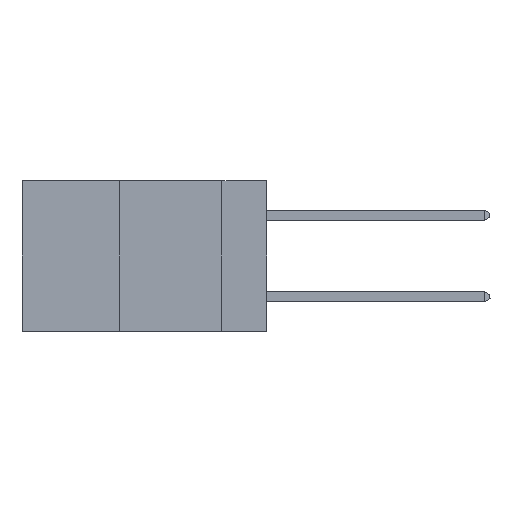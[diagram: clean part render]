
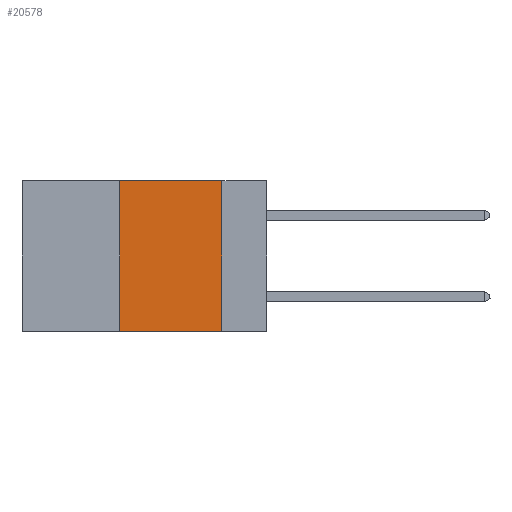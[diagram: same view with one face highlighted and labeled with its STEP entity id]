
A CAD part, left-side view. The second image highlights one B-rep face of the part: STEP entity #20578.
In plain terms, the highlighted planar face has unit normal (-1, 0, 0).
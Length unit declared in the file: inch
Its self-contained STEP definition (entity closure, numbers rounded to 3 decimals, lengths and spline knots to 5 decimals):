
#729 = VECTOR ( 'NONE', #40134, 39.37008 ) ;
#1886 = DIRECTION ( 'NONE',  ( 1., 0., 0. ) ) ;
#1929 = ORIENTED_EDGE ( 'NONE', *, *, #42733, .F. ) ;
#3078 = DIRECTION ( 'NONE',  ( 0., 0., 1. ) ) ;
#4590 = CARTESIAN_POINT ( 'NONE',  ( 0., 0.11, 0. ) ) ;
#6952 = FACE_OUTER_BOUND ( 'NONE', #26723, .T. ) ;
#14040 = EDGE_CURVE ( 'NONE', #44222, #44267, #23990, .T. ) ;
#16548 = PLANE ( 'NONE',  #31509 ) ;
#16716 = CARTESIAN_POINT ( 'NONE',  ( 0., 0.36, -0.37 ) ) ;
#18320 = DIRECTION ( 'NONE',  ( 0., 0., -1. ) ) ;
#20578 = ADVANCED_FACE ( 'NONE', ( #6952 ), #16548, .F. ) ;
#22986 = VERTEX_POINT ( 'NONE', #32735 ) ;
#23944 = VECTOR ( 'NONE', #18320, 39.37008 ) ;
#23990 = LINE ( 'NONE', #35572, #23944 ) ;
#25432 = CARTESIAN_POINT ( 'NONE',  ( 0., 0.6, 0. ) ) ;
#26349 = CARTESIAN_POINT ( 'NONE',  ( 0., 0.6, -0.37 ) ) ;
#26723 = EDGE_LOOP ( 'NONE', ( #32185, #44638, #1929, #27105 ) ) ;
#27105 = ORIENTED_EDGE ( 'NONE', *, *, #38295, .T. ) ;
#27299 = DIRECTION ( 'NONE',  ( 0., 0., -1. ) ) ;
#29569 = LINE ( 'NONE', #26349, #729 ) ;
#29878 = CARTESIAN_POINT ( 'NONE',  ( 0., 0.11, -0.37 ) ) ;
#30249 = VERTEX_POINT ( 'NONE', #16716 ) ;
#31509 = AXIS2_PLACEMENT_3D ( 'NONE', #33338, #1886, #27299 ) ;
#31716 = CARTESIAN_POINT ( 'NONE',  ( 0., 0.36, 0. ) ) ;
#32185 = ORIENTED_EDGE ( 'NONE', *, *, #14040, .F. ) ;
#32242 = DIRECTION ( 'NONE',  ( 0., -1., 0. ) ) ;
#32735 = CARTESIAN_POINT ( 'NONE',  ( 0., 0.36, 0. ) ) ;
#33338 = CARTESIAN_POINT ( 'NONE',  ( 0., 0.6, 0. ) ) ;
#33484 = LINE ( 'NONE', #25432, #40369 ) ;
#34177 = LINE ( 'NONE', #31716, #42093 ) ;
#35572 = CARTESIAN_POINT ( 'NONE',  ( 0., 0.11, 0. ) ) ;
#38295 = EDGE_CURVE ( 'NONE', #30249, #44267, #29569, .T. ) ;
#40134 = DIRECTION ( 'NONE',  ( 0., -1., 0. ) ) ;
#40369 = VECTOR ( 'NONE', #32242, 39.37008 ) ;
#42093 = VECTOR ( 'NONE', #3078, 39.37008 ) ;
#42733 = EDGE_CURVE ( 'NONE', #30249, #22986, #34177, .T. ) ;
#44222 = VERTEX_POINT ( 'NONE', #4590 ) ;
#44267 = VERTEX_POINT ( 'NONE', #29878 ) ;
#44638 = ORIENTED_EDGE ( 'NONE', *, *, #45264, .F. ) ;
#45264 = EDGE_CURVE ( 'NONE', #22986, #44222, #33484, .T. ) ;
